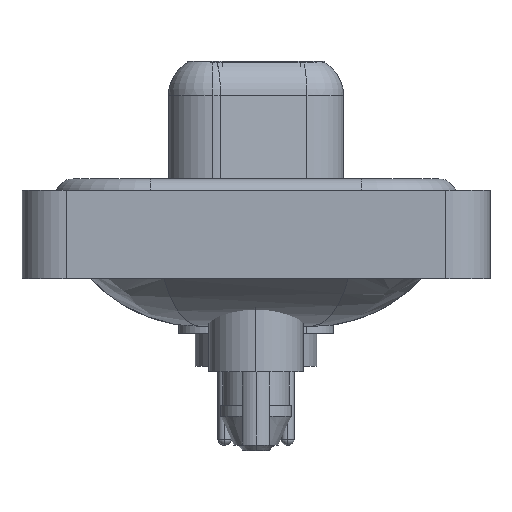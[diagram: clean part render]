
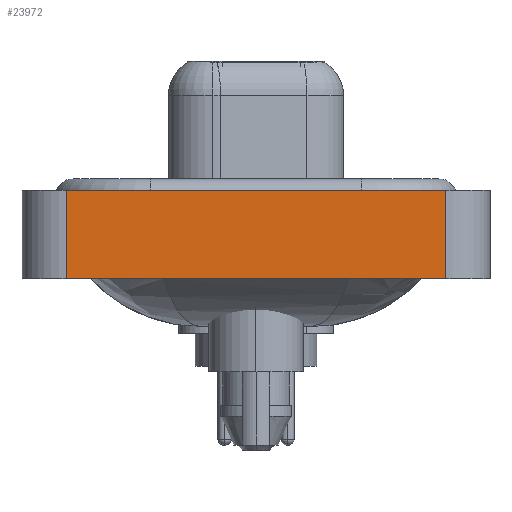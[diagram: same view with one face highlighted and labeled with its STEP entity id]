
A CAD part, left-side view. The second image highlights one B-rep face of the part: STEP entity #23972.
In plain terms, the highlighted planar face has unit normal (-1, 0, 0).
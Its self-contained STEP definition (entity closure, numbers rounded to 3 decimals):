
#266 = DIRECTION ( 'NONE',  ( 0., 0., 1. ) ) ;
#528 = EDGE_CURVE ( 'NONE', #6369, #1758, #10246, .T. ) ;
#1758 = VERTEX_POINT ( 'NONE', #19375 ) ;
#3006 = VECTOR ( 'NONE', #3532, 1000. ) ;
#3532 = DIRECTION ( 'NONE',  ( 0., -1., 0. ) ) ;
#3660 = DIRECTION ( 'NONE',  ( 0., -1., 0. ) ) ;
#3926 = EDGE_CURVE ( 'NONE', #20995, #11349, #8419, .T. ) ;
#4064 = AXIS2_PLACEMENT_3D ( 'NONE', #23243, #5752, #266 ) ;
#5623 = FACE_OUTER_BOUND ( 'NONE', #12798, .T. ) ;
#5752 = DIRECTION ( 'NONE',  ( -1., 0., 0. ) ) ;
#5787 = ORIENTED_EDGE ( 'NONE', *, *, #528, .F. ) ;
#6255 = ORIENTED_EDGE ( 'NONE', *, *, #7333, .F. ) ;
#6369 = VERTEX_POINT ( 'NONE', #8039 ) ;
#6415 = CARTESIAN_POINT ( 'NONE',  ( -7.35, 8.55, -3.6 ) ) ;
#7069 = ORIENTED_EDGE ( 'NONE', *, *, #3926, .T. ) ;
#7333 = EDGE_CURVE ( 'NONE', #1758, #11349, #13857, .T. ) ;
#8039 = CARTESIAN_POINT ( 'NONE',  ( -7.35, 8.55, -3.6 ) ) ;
#8419 = LINE ( 'NONE', #12509, #9729 ) ;
#9729 = VECTOR ( 'NONE', #16216, 1000. ) ;
#10246 = LINE ( 'NONE', #6415, #13290 ) ;
#10649 = ORIENTED_EDGE ( 'NONE', *, *, #22516, .T. ) ;
#10939 = LINE ( 'NONE', #18990, #3006 ) ;
#11349 = VERTEX_POINT ( 'NONE', #22228 ) ;
#11410 = VECTOR ( 'NONE', #3660, 1000. ) ;
#12509 = CARTESIAN_POINT ( 'NONE',  ( -7.35, -8.55, -3.6 ) ) ;
#12798 = EDGE_LOOP ( 'NONE', ( #7069, #6255, #5787, #10649 ) ) ;
#13290 = VECTOR ( 'NONE', #14188, 1000. ) ;
#13405 = PLANE ( 'NONE',  #4064 ) ;
#13857 = LINE ( 'NONE', #19750, #11410 ) ;
#14188 = DIRECTION ( 'NONE',  ( 0., 0., 1. ) ) ;
#16216 = DIRECTION ( 'NONE',  ( 0., 0., 1. ) ) ;
#17850 = CARTESIAN_POINT ( 'NONE',  ( -7.35, -8.55, -3.6 ) ) ;
#18990 = CARTESIAN_POINT ( 'NONE',  ( -7.35, -8.55, -3.6 ) ) ;
#19375 = CARTESIAN_POINT ( 'NONE',  ( -7.35, 8.55, 0.4 ) ) ;
#19750 = CARTESIAN_POINT ( 'NONE',  ( -7.35, -8.55, 0.4 ) ) ;
#20995 = VERTEX_POINT ( 'NONE', #17850 ) ;
#22228 = CARTESIAN_POINT ( 'NONE',  ( -7.35, -8.55, 0.4 ) ) ;
#22516 = EDGE_CURVE ( 'NONE', #6369, #20995, #10939, .T. ) ;
#23243 = CARTESIAN_POINT ( 'NONE',  ( -7.35, -8.55, -3.6 ) ) ;
#23972 = ADVANCED_FACE ( 'NONE', ( #5623 ), #13405, .T. ) ;
